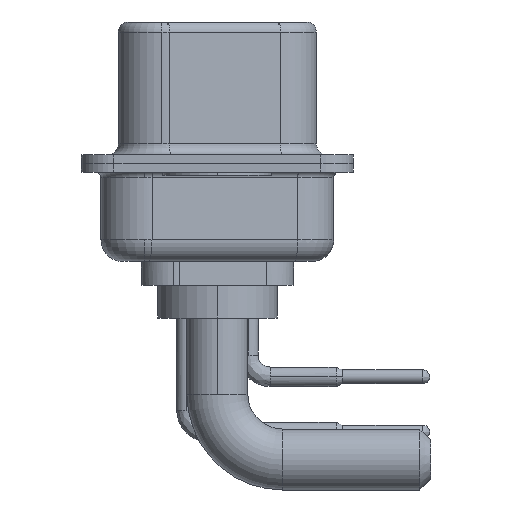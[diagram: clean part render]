
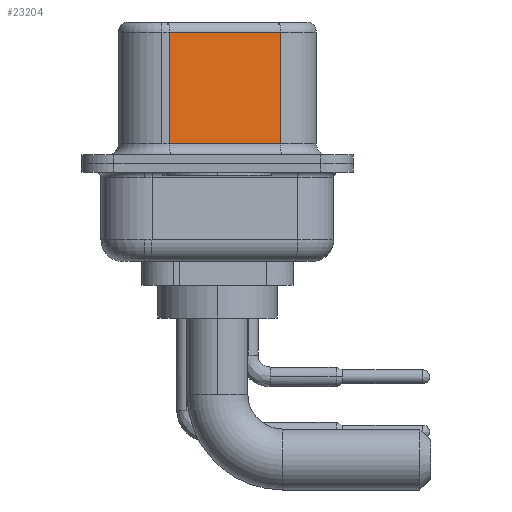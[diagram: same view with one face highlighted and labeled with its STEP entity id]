
A CAD part, left-side view. The second image highlights one B-rep face of the part: STEP entity #23204.
In plain terms, the highlighted planar face has unit normal (-0.985, -0.174, 0).
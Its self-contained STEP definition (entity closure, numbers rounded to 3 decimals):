
#647 = CARTESIAN_POINT ( 'NONE',  ( 4.58, -2.897, 6.52 ) ) ;
#851 = VERTEX_POINT ( 'NONE', #11518 ) ;
#2955 = LINE ( 'NONE', #13942, #5789 ) ;
#3167 = DIRECTION ( 'NONE',  ( 0.985, 0.174, 0. ) ) ;
#4138 = CARTESIAN_POINT ( 'NONE',  ( 3.68, 2.203, 6.52 ) ) ;
#4607 = VERTEX_POINT ( 'NONE', #21344 ) ;
#4764 = VECTOR ( 'NONE', #8353, 1000. ) ;
#5789 = VECTOR ( 'NONE', #21273, 1000. ) ;
#6339 = EDGE_CURVE ( 'NONE', #4607, #12429, #7987, .T. ) ;
#6892 = PLANE ( 'NONE',  #13649 ) ;
#7835 = EDGE_CURVE ( 'NONE', #14555, #851, #11735, .T. ) ;
#7987 = LINE ( 'NONE', #4138, #17439 ) ;
#8311 = CARTESIAN_POINT ( 'NONE',  ( 3.68, 2.203, 0.9 ) ) ;
#8353 = DIRECTION ( 'NONE',  ( 0., 0., -1. ) ) ;
#8725 = ORIENTED_EDGE ( 'NONE', *, *, #6339, .T. ) ;
#9920 = CARTESIAN_POINT ( 'NONE',  ( 4.58, -2.897, 0.9 ) ) ;
#10857 = FACE_OUTER_BOUND ( 'NONE', #13420, .T. ) ;
#11515 = ORIENTED_EDGE ( 'NONE', *, *, #18119, .T. ) ;
#11518 = CARTESIAN_POINT ( 'NONE',  ( 4.58, -2.897, 0.9 ) ) ;
#11724 = LINE ( 'NONE', #9920, #19980 ) ;
#11735 = LINE ( 'NONE', #647, #4764 ) ;
#12429 = VERTEX_POINT ( 'NONE', #8311 ) ;
#13420 = EDGE_LOOP ( 'NONE', ( #20670, #20090, #8725, #11515 ) ) ;
#13649 = AXIS2_PLACEMENT_3D ( 'NONE', #18338, #3167, #18216 ) ;
#13942 = CARTESIAN_POINT ( 'NONE',  ( 4.58, -2.897, 6.02 ) ) ;
#14555 = VERTEX_POINT ( 'NONE', #17189 ) ;
#14985 = DIRECTION ( 'NONE',  ( 0.174, -0.985, 0. ) ) ;
#17030 = DIRECTION ( 'NONE',  ( 0., 0., -1. ) ) ;
#17189 = CARTESIAN_POINT ( 'NONE',  ( 4.58, -2.897, 6.02 ) ) ;
#17439 = VECTOR ( 'NONE', #17030, 1000. ) ;
#18119 = EDGE_CURVE ( 'NONE', #12429, #851, #11724, .T. ) ;
#18216 = DIRECTION ( 'NONE',  ( -0.174, 0.985, 0. ) ) ;
#18338 = CARTESIAN_POINT ( 'NONE',  ( 4.58, -2.897, 6.52 ) ) ;
#19980 = VECTOR ( 'NONE', #14985, 1000. ) ;
#20090 = ORIENTED_EDGE ( 'NONE', *, *, #21046, .T. ) ;
#20670 = ORIENTED_EDGE ( 'NONE', *, *, #7835, .F. ) ;
#21046 = EDGE_CURVE ( 'NONE', #14555, #4607, #2955, .T. ) ;
#21273 = DIRECTION ( 'NONE',  ( -0.174, 0.985, 0. ) ) ;
#21344 = CARTESIAN_POINT ( 'NONE',  ( 3.68, 2.203, 6.02 ) ) ;
#23204 = ADVANCED_FACE ( 'NONE', ( #10857 ), #6892, .F. ) ;
